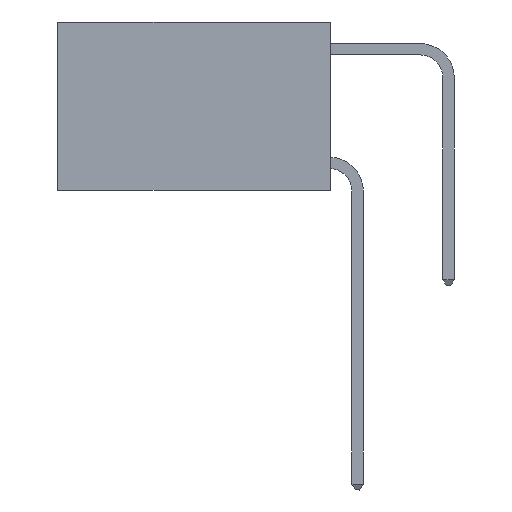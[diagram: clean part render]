
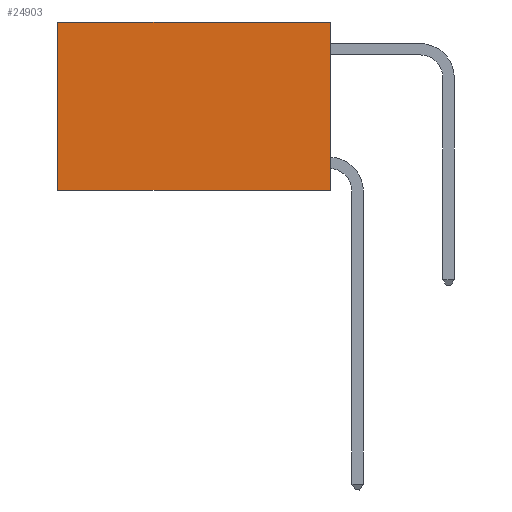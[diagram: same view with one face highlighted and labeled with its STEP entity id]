
A CAD part, left-side view. The second image highlights one B-rep face of the part: STEP entity #24903.
In plain terms, the highlighted planar face has unit normal (-1, 0, 0).
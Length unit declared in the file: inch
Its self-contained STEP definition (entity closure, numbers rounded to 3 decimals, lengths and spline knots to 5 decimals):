
#220 = ORIENTED_EDGE ( 'NONE', *, *, #14648, .T. ) ;
#873 = EDGE_CURVE ( 'NONE', #18758, #25273, #13969, .T. ) ;
#945 = AXIS2_PLACEMENT_3D ( 'NONE', #22195, #22035, #1422 ) ;
#1076 = VERTEX_POINT ( 'NONE', #28420 ) ;
#1422 = DIRECTION ( 'NONE',  ( 0., 0., -1. ) ) ;
#1459 = VERTEX_POINT ( 'NONE', #3305 ) ;
#2473 = CARTESIAN_POINT ( 'NONE',  ( 0.2625, 0., -0.37 ) ) ;
#3305 = CARTESIAN_POINT ( 'NONE',  ( 0.2625, 0.6, 0. ) ) ;
#3658 = CARTESIAN_POINT ( 'NONE',  ( 0.2625, 0., 0. ) ) ;
#4173 = VECTOR ( 'NONE', #7769, 39.37008 ) ;
#5030 = DIRECTION ( 'NONE',  ( 0., 1., 0. ) ) ;
#6340 = EDGE_CURVE ( 'NONE', #1076, #1459, #24467, .T. ) ;
#7467 = LINE ( 'NONE', #23886, #4173 ) ;
#7769 = DIRECTION ( 'NONE',  ( 0., 0., -1. ) ) ;
#8341 = LINE ( 'NONE', #24458, #18232 ) ;
#10352 = VECTOR ( 'NONE', #12898, 39.37008 ) ;
#11038 = EDGE_LOOP ( 'NONE', ( #220, #17498, #18249, #15385 ) ) ;
#12371 = CARTESIAN_POINT ( 'NONE',  ( 0.2625, 0., -0.37 ) ) ;
#12401 = VECTOR ( 'NONE', #5030, 39.37008 ) ;
#12898 = DIRECTION ( 'NONE',  ( 0., 1., 0. ) ) ;
#12907 = FACE_OUTER_BOUND ( 'NONE', #11038, .T. ) ;
#13969 = LINE ( 'NONE', #2473, #12401 ) ;
#14648 = EDGE_CURVE ( 'NONE', #1459, #25273, #7467, .T. ) ;
#15213 = EDGE_CURVE ( 'NONE', #1076, #18758, #8341, .T. ) ;
#15385 = ORIENTED_EDGE ( 'NONE', *, *, #6340, .T. ) ;
#17498 = ORIENTED_EDGE ( 'NONE', *, *, #873, .F. ) ;
#17620 = PLANE ( 'NONE',  #945 ) ;
#18232 = VECTOR ( 'NONE', #19576, 39.37008 ) ;
#18249 = ORIENTED_EDGE ( 'NONE', *, *, #15213, .F. ) ;
#18758 = VERTEX_POINT ( 'NONE', #12371 ) ;
#19576 = DIRECTION ( 'NONE',  ( 0., 0., -1. ) ) ;
#19863 = CARTESIAN_POINT ( 'NONE',  ( 0.2625, 0.6, -0.37 ) ) ;
#22035 = DIRECTION ( 'NONE',  ( 1., 0., 0. ) ) ;
#22195 = CARTESIAN_POINT ( 'NONE',  ( 0.2625, 0., 0. ) ) ;
#23886 = CARTESIAN_POINT ( 'NONE',  ( 0.2625, 0.6, 0. ) ) ;
#24458 = CARTESIAN_POINT ( 'NONE',  ( 0.2625, 0., 0. ) ) ;
#24467 = LINE ( 'NONE', #3658, #10352 ) ;
#24903 = ADVANCED_FACE ( 'NONE', ( #12907 ), #17620, .F. ) ;
#25273 = VERTEX_POINT ( 'NONE', #19863 ) ;
#28420 = CARTESIAN_POINT ( 'NONE',  ( 0.2625, 0., 0. ) ) ;
